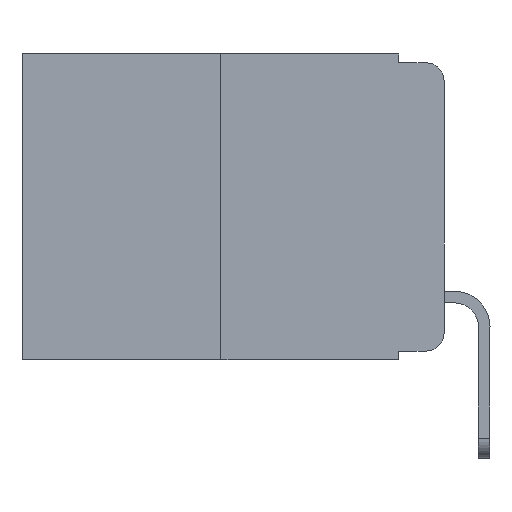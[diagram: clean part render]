
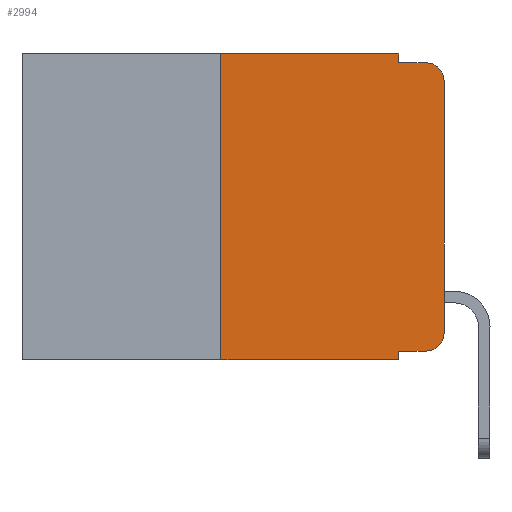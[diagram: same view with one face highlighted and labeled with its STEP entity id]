
A CAD part, left-side view. The second image highlights one B-rep face of the part: STEP entity #2994.
In plain terms, the highlighted planar face has unit normal (-1, 0, 0).
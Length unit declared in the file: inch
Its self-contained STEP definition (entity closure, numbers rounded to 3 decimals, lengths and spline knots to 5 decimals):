
#338 = VECTOR ( 'NONE', #1582, 39.37008 ) ;
#619 = ORIENTED_EDGE ( 'NONE', *, *, #5154, .F. ) ;
#774 = ORIENTED_EDGE ( 'NONE', *, *, #10476, .F. ) ;
#972 = CARTESIAN_POINT ( 'NONE',  ( 0., 0.051, -0.01 ) ) ;
#1113 = CARTESIAN_POINT ( 'NONE',  ( 0., 0.473, 0. ) ) ;
#1177 = LINE ( 'NONE', #7226, #7665 ) ;
#1279 = LINE ( 'NONE', #9299, #2882 ) ;
#1459 = EDGE_CURVE ( 'NONE', #15980, #12603, #3156, .T. ) ;
#1582 = DIRECTION ( 'NONE',  ( 0., 0., -1. ) ) ;
#1800 = LINE ( 'NONE', #1113, #2743 ) ;
#1944 = DIRECTION ( 'NONE',  ( -1., 0., 0. ) ) ;
#1989 = EDGE_LOOP ( 'NONE', ( #10243, #6139, #19081, #16730, #774, #619, #18417, #11443, #6297, #2401 ) ) ;
#2104 = EDGE_CURVE ( 'NONE', #7997, #5262, #4745, .T. ) ;
#2132 = EDGE_CURVE ( 'NONE', #6714, #5262, #17090, .T. ) ;
#2311 = EDGE_CURVE ( 'NONE', #14451, #12583, #1279, .T. ) ;
#2401 = ORIENTED_EDGE ( 'NONE', *, *, #4966, .T. ) ;
#2743 = VECTOR ( 'NONE', #19101, 39.37008 ) ;
#2882 = VECTOR ( 'NONE', #3262, 39.37008 ) ;
#2901 = AXIS2_PLACEMENT_3D ( 'NONE', #9323, #6649, #4967 ) ;
#2994 = ADVANCED_FACE ( 'NONE', ( #16122 ), #18373, .F. ) ;
#3156 = LINE ( 'NONE', #12568, #10560 ) ;
#3262 = DIRECTION ( 'NONE',  ( 0., 0., -1. ) ) ;
#3265 = CIRCLE ( 'NONE', #5210, 0.02 ) ;
#3691 = EDGE_CURVE ( 'NONE', #7997, #10062, #15860, .T. ) ;
#3786 = CARTESIAN_POINT ( 'NONE',  ( 0., 0.051, -0.333 ) ) ;
#3921 = CARTESIAN_POINT ( 'NONE',  ( 0., 0., -0.313 ) ) ;
#4739 = DIRECTION ( 'NONE',  ( 0., 0., -1. ) ) ;
#4745 = LINE ( 'NONE', #8799, #338 ) ;
#4966 = EDGE_CURVE ( 'NONE', #10062, #15980, #3265, .T. ) ;
#4967 = DIRECTION ( 'NONE',  ( 0., 0., -1. ) ) ;
#5154 = EDGE_CURVE ( 'NONE', #6714, #10230, #1177, .T. ) ;
#5188 = DIRECTION ( 'NONE',  ( 0., -1., 0. ) ) ;
#5210 = AXIS2_PLACEMENT_3D ( 'NONE', #10871, #1944, #4739 ) ;
#5223 = CARTESIAN_POINT ( 'NONE',  ( 0., 0.051, 0. ) ) ;
#5262 = VERTEX_POINT ( 'NONE', #18578 ) ;
#5612 = VECTOR ( 'NONE', #12879, 39.37008 ) ;
#5836 = CARTESIAN_POINT ( 'NONE',  ( 0., 0., -0.03 ) ) ;
#6139 = ORIENTED_EDGE ( 'NONE', *, *, #9259, .T. ) ;
#6297 = ORIENTED_EDGE ( 'NONE', *, *, #3691, .T. ) ;
#6610 = DIRECTION ( 'NONE',  ( 0., 0., -1. ) ) ;
#6649 = DIRECTION ( 'NONE',  ( -1., 0., 0. ) ) ;
#6714 = VERTEX_POINT ( 'NONE', #13637 ) ;
#7226 = CARTESIAN_POINT ( 'NONE',  ( 0., 0.25, 0. ) ) ;
#7665 = VECTOR ( 'NONE', #13192, 39.37008 ) ;
#7771 = VERTEX_POINT ( 'NONE', #16285 ) ;
#7997 = VERTEX_POINT ( 'NONE', #3786 ) ;
#8799 = CARTESIAN_POINT ( 'NONE',  ( 0., 0.051, 0. ) ) ;
#9191 = VECTOR ( 'NONE', #5188, 39.37008 ) ;
#9259 = EDGE_CURVE ( 'NONE', #12603, #7771, #16734, .T. ) ;
#9299 = CARTESIAN_POINT ( 'NONE',  ( 0., 0.051, 0. ) ) ;
#9323 = CARTESIAN_POINT ( 'NONE',  ( 0., 0.02, -0.03 ) ) ;
#9815 = CARTESIAN_POINT ( 'NONE',  ( 0., 0.051, -0.333 ) ) ;
#10062 = VERTEX_POINT ( 'NONE', #18128 ) ;
#10230 = VERTEX_POINT ( 'NONE', #18253 ) ;
#10243 = ORIENTED_EDGE ( 'NONE', *, *, #1459, .T. ) ;
#10476 = EDGE_CURVE ( 'NONE', #10230, #14451, #1800, .T. ) ;
#10560 = VECTOR ( 'NONE', #18551, 39.37008 ) ;
#10871 = CARTESIAN_POINT ( 'NONE',  ( 0., 0.02, -0.313 ) ) ;
#11213 = VECTOR ( 'NONE', #13210, 39.37008 ) ;
#11443 = ORIENTED_EDGE ( 'NONE', *, *, #2104, .F. ) ;
#11503 = LINE ( 'NONE', #972, #9191 ) ;
#11902 = AXIS2_PLACEMENT_3D ( 'NONE', #15586, #14206, #6610 ) ;
#12303 = EDGE_CURVE ( 'NONE', #12583, #7771, #11503, .T. ) ;
#12568 = CARTESIAN_POINT ( 'NONE',  ( 0., 0., 0. ) ) ;
#12583 = VERTEX_POINT ( 'NONE', #13421 ) ;
#12603 = VERTEX_POINT ( 'NONE', #5836 ) ;
#12879 = DIRECTION ( 'NONE',  ( 0., -1., 0. ) ) ;
#13192 = DIRECTION ( 'NONE',  ( 0., 0., 1. ) ) ;
#13210 = DIRECTION ( 'NONE',  ( 0., -1., 0. ) ) ;
#13421 = CARTESIAN_POINT ( 'NONE',  ( 0., 0.051, -0.01 ) ) ;
#13637 = CARTESIAN_POINT ( 'NONE',  ( 0., 0.25, -0.343 ) ) ;
#14206 = DIRECTION ( 'NONE',  ( 1., 0., 0. ) ) ;
#14451 = VERTEX_POINT ( 'NONE', #5223 ) ;
#15586 = CARTESIAN_POINT ( 'NONE',  ( 0., 0.473, 0. ) ) ;
#15860 = LINE ( 'NONE', #9815, #5612 ) ;
#15980 = VERTEX_POINT ( 'NONE', #3921 ) ;
#16122 = FACE_OUTER_BOUND ( 'NONE', #1989, .T. ) ;
#16285 = CARTESIAN_POINT ( 'NONE',  ( 0., 0.02, -0.01 ) ) ;
#16339 = CARTESIAN_POINT ( 'NONE',  ( 0., 0.473, -0.343 ) ) ;
#16730 = ORIENTED_EDGE ( 'NONE', *, *, #2311, .F. ) ;
#16734 = CIRCLE ( 'NONE', #2901, 0.02 ) ;
#17090 = LINE ( 'NONE', #16339, #11213 ) ;
#18128 = CARTESIAN_POINT ( 'NONE',  ( 0., 0.02, -0.333 ) ) ;
#18253 = CARTESIAN_POINT ( 'NONE',  ( 0., 0.25, 0. ) ) ;
#18373 = PLANE ( 'NONE',  #11902 ) ;
#18417 = ORIENTED_EDGE ( 'NONE', *, *, #2132, .T. ) ;
#18551 = DIRECTION ( 'NONE',  ( 0., 0., 1. ) ) ;
#18578 = CARTESIAN_POINT ( 'NONE',  ( 0., 0.051, -0.343 ) ) ;
#19081 = ORIENTED_EDGE ( 'NONE', *, *, #12303, .F. ) ;
#19101 = DIRECTION ( 'NONE',  ( 0., -1., 0. ) ) ;
